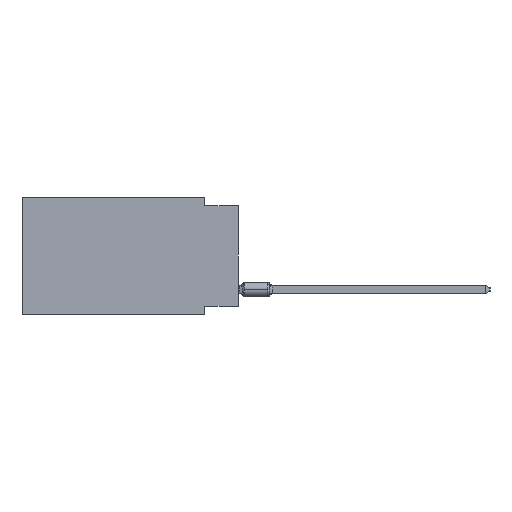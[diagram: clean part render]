
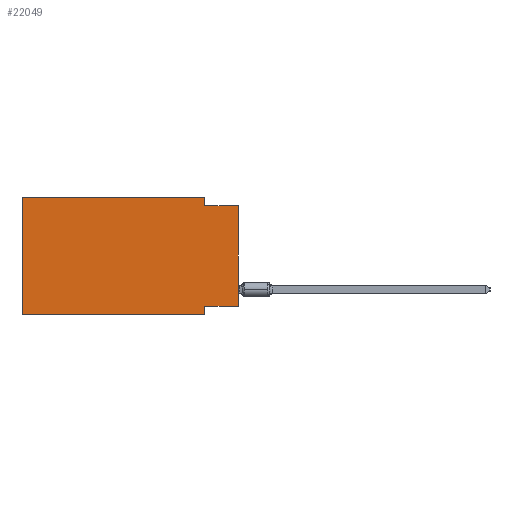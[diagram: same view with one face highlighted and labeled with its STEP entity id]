
A CAD part, left-side view. The second image highlights one B-rep face of the part: STEP entity #22049.
In plain terms, the highlighted planar face has unit normal (-1, 0, 0).
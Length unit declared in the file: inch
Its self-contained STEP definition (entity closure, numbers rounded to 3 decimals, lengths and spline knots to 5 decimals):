
#247 = EDGE_CURVE ( 'NONE', #28619, #16569, #478, .T. ) ;
#261 = VECTOR ( 'NONE', #31430, 39.37008 ) ;
#478 = LINE ( 'NONE', #5183, #1070 ) ;
#606 = CARTESIAN_POINT ( 'NONE',  ( 0., 0., -0.025 ) ) ;
#614 = FACE_OUTER_BOUND ( 'NONE', #18784, .T. ) ;
#778 = CARTESIAN_POINT ( 'NONE',  ( 0., 0.645, 0. ) ) ;
#955 = CARTESIAN_POINT ( 'NONE',  ( 0., 0., -0.325 ) ) ;
#1070 = VECTOR ( 'NONE', #24950, 39.37008 ) ;
#1731 = ORIENTED_EDGE ( 'NONE', *, *, #31536, .T. ) ;
#2152 = VECTOR ( 'NONE', #13603, 39.37008 ) ;
#4432 = VERTEX_POINT ( 'NONE', #955 ) ;
#5057 = DIRECTION ( 'NONE',  ( 0., -1., 0. ) ) ;
#5183 = CARTESIAN_POINT ( 'NONE',  ( 0., 0.1, -0.35 ) ) ;
#5219 = AXIS2_PLACEMENT_3D ( 'NONE', #778, #30413, #12755 ) ;
#5420 = LINE ( 'NONE', #25310, #6961 ) ;
#6391 = EDGE_CURVE ( 'NONE', #30731, #21030, #30443, .T. ) ;
#6933 = DIRECTION ( 'NONE',  ( 0., -1., 0. ) ) ;
#6961 = VECTOR ( 'NONE', #10427, 39.37008 ) ;
#8083 = PLANE ( 'NONE',  #5219 ) ;
#9002 = EDGE_CURVE ( 'NONE', #21030, #25693, #20567, .T. ) ;
#9631 = CARTESIAN_POINT ( 'NONE',  ( 0., 0.1, -0.025 ) ) ;
#10205 = VECTOR ( 'NONE', #16188, 39.37008 ) ;
#10275 = ORIENTED_EDGE ( 'NONE', *, *, #18716, .F. ) ;
#10393 = ORIENTED_EDGE ( 'NONE', *, *, #21009, .F. ) ;
#10427 = DIRECTION ( 'NONE',  ( 0., 1., 0. ) ) ;
#10474 = VERTEX_POINT ( 'NONE', #9631 ) ;
#11034 = LINE ( 'NONE', #28687, #261 ) ;
#12172 = CARTESIAN_POINT ( 'NONE',  ( 0., 0.1, 0. ) ) ;
#12755 = DIRECTION ( 'NONE',  ( 0., 0., -1. ) ) ;
#13147 = VERTEX_POINT ( 'NONE', #606 ) ;
#13603 = DIRECTION ( 'NONE',  ( 0., -1., 0. ) ) ;
#14543 = EDGE_CURVE ( 'NONE', #4432, #28619, #5420, .T. ) ;
#14669 = ORIENTED_EDGE ( 'NONE', *, *, #247, .F. ) ;
#15273 = EDGE_CURVE ( 'NONE', #4432, #13147, #11034, .T. ) ;
#15855 = CARTESIAN_POINT ( 'NONE',  ( 0., 0.645, 0. ) ) ;
#16188 = DIRECTION ( 'NONE',  ( 0., 0., 1. ) ) ;
#16569 = VERTEX_POINT ( 'NONE', #19292 ) ;
#16797 = CARTESIAN_POINT ( 'NONE',  ( 0., 0., -0.025 ) ) ;
#17070 = CARTESIAN_POINT ( 'NONE',  ( 0., 0.1, 0. ) ) ;
#18716 = EDGE_CURVE ( 'NONE', #25693, #10474, #24680, .T. ) ;
#18784 = EDGE_LOOP ( 'NONE', ( #26715, #10393, #10275, #25592, #25694, #1731, #14669, #27968 ) ) ;
#19292 = CARTESIAN_POINT ( 'NONE',  ( 0., 0.1, -0.35 ) ) ;
#19397 = LINE ( 'NONE', #16797, #30490 ) ;
#19812 = LINE ( 'NONE', #29692, #27463 ) ;
#20415 = CARTESIAN_POINT ( 'NONE',  ( 0., 0.645, 0. ) ) ;
#20567 = LINE ( 'NONE', #20415, #2152 ) ;
#21009 = EDGE_CURVE ( 'NONE', #10474, #13147, #19397, .T. ) ;
#21030 = VERTEX_POINT ( 'NONE', #21979 ) ;
#21979 = CARTESIAN_POINT ( 'NONE',  ( 0., 0.645, 0. ) ) ;
#22049 = ADVANCED_FACE ( 'NONE', ( #614 ), #8083, .F. ) ;
#22601 = CARTESIAN_POINT ( 'NONE',  ( 0., 0.645, -0.35 ) ) ;
#24680 = LINE ( 'NONE', #17070, #26979 ) ;
#24950 = DIRECTION ( 'NONE',  ( 0., 0., -1. ) ) ;
#25310 = CARTESIAN_POINT ( 'NONE',  ( 0., 0., -0.325 ) ) ;
#25592 = ORIENTED_EDGE ( 'NONE', *, *, #9002, .F. ) ;
#25693 = VERTEX_POINT ( 'NONE', #12172 ) ;
#25694 = ORIENTED_EDGE ( 'NONE', *, *, #6391, .F. ) ;
#26715 = ORIENTED_EDGE ( 'NONE', *, *, #15273, .T. ) ;
#26979 = VECTOR ( 'NONE', #31835, 39.37008 ) ;
#27463 = VECTOR ( 'NONE', #5057, 39.37008 ) ;
#27968 = ORIENTED_EDGE ( 'NONE', *, *, #14543, .F. ) ;
#28619 = VERTEX_POINT ( 'NONE', #29498 ) ;
#28687 = CARTESIAN_POINT ( 'NONE',  ( 0., 0., 0. ) ) ;
#29498 = CARTESIAN_POINT ( 'NONE',  ( 0., 0.1, -0.325 ) ) ;
#29692 = CARTESIAN_POINT ( 'NONE',  ( 0., 0.645, -0.35 ) ) ;
#30413 = DIRECTION ( 'NONE',  ( 1., 0., 0. ) ) ;
#30443 = LINE ( 'NONE', #15855, #10205 ) ;
#30490 = VECTOR ( 'NONE', #6933, 39.37008 ) ;
#30731 = VERTEX_POINT ( 'NONE', #22601 ) ;
#31430 = DIRECTION ( 'NONE',  ( 0., 0., 1. ) ) ;
#31536 = EDGE_CURVE ( 'NONE', #30731, #16569, #19812, .T. ) ;
#31835 = DIRECTION ( 'NONE',  ( 0., 0., -1. ) ) ;
